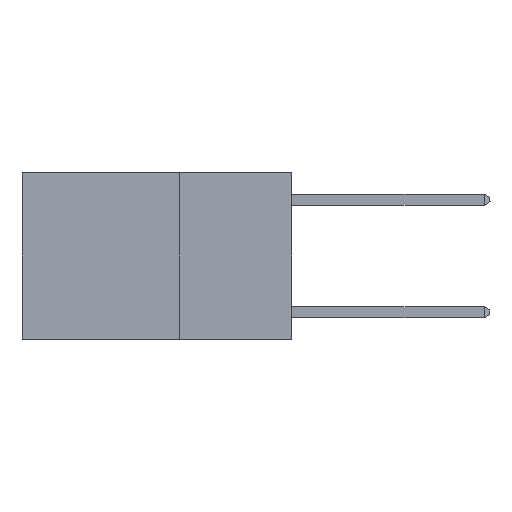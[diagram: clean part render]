
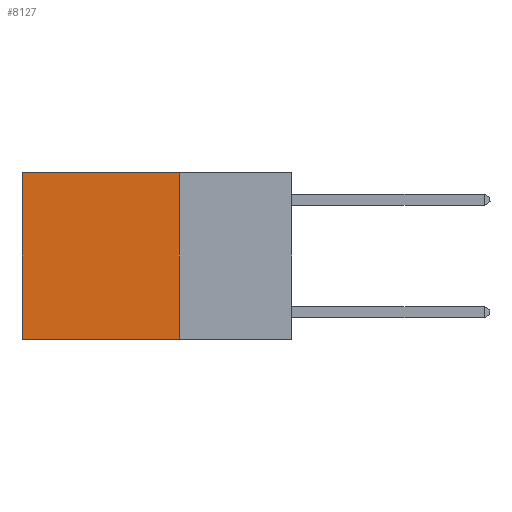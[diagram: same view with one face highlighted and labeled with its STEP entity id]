
A CAD part, left-side view. The second image highlights one B-rep face of the part: STEP entity #8127.
In plain terms, the highlighted planar face has unit normal (-1, 0, 0).
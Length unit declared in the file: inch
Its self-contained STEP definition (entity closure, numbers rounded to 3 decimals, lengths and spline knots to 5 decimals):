
#13 = CARTESIAN_POINT ( 'NONE',  ( 0.2625, 0.25, -0.37 ) ) ;
#69 = VERTEX_POINT ( 'NONE', #13 ) ;
#527 = CARTESIAN_POINT ( 'NONE',  ( 0.2625, 0.25, 0. ) ) ;
#608 = ORIENTED_EDGE ( 'NONE', *, *, #3062, .T. ) ;
#844 = EDGE_LOOP ( 'NONE', ( #2182, #7662, #9152, #608 ) ) ;
#1154 = VECTOR ( 'NONE', #4065, 39.37008 ) ;
#1278 = DIRECTION ( 'NONE',  ( 1., 0., 0. ) ) ;
#1807 = VECTOR ( 'NONE', #4570, 39.37008 ) ;
#2123 = CARTESIAN_POINT ( 'NONE',  ( 0.2625, 0.6, 0. ) ) ;
#2182 = ORIENTED_EDGE ( 'NONE', *, *, #4545, .T. ) ;
#2371 = CARTESIAN_POINT ( 'NONE',  ( 0.2625, 0.6, -0.37 ) ) ;
#2386 = FACE_OUTER_BOUND ( 'NONE', #844, .T. ) ;
#2499 = EDGE_CURVE ( 'NONE', #5500, #69, #8666, .T. ) ;
#3062 = EDGE_CURVE ( 'NONE', #5500, #7099, #7307, .T. ) ;
#4065 = DIRECTION ( 'NONE',  ( 0., 0., -1. ) ) ;
#4492 = PLANE ( 'NONE',  #6735 ) ;
#4545 = EDGE_CURVE ( 'NONE', #7099, #7263, #8053, .T. ) ;
#4570 = DIRECTION ( 'NONE',  ( 0., 1., 0. ) ) ;
#4842 = CARTESIAN_POINT ( 'NONE',  ( 0.2625, 0.25, 0. ) ) ;
#5004 = EDGE_CURVE ( 'NONE', #69, #7263, #7740, .T. ) ;
#5500 = VERTEX_POINT ( 'NONE', #9041 ) ;
#5644 = VECTOR ( 'NONE', #6610, 39.37008 ) ;
#5980 = CARTESIAN_POINT ( 'NONE',  ( 0.2625, 0.25, 0. ) ) ;
#6012 = CARTESIAN_POINT ( 'NONE',  ( 0.2625, 0.6, 0. ) ) ;
#6382 = VECTOR ( 'NONE', #7897, 39.37008 ) ;
#6522 = DIRECTION ( 'NONE',  ( 0., 0., -1. ) ) ;
#6610 = DIRECTION ( 'NONE',  ( 0., 1., 0. ) ) ;
#6735 = AXIS2_PLACEMENT_3D ( 'NONE', #527, #1278, #6522 ) ;
#7099 = VERTEX_POINT ( 'NONE', #2123 ) ;
#7174 = CARTESIAN_POINT ( 'NONE',  ( 0.2625, 0.25, -0.37 ) ) ;
#7263 = VERTEX_POINT ( 'NONE', #2371 ) ;
#7307 = LINE ( 'NONE', #5980, #5644 ) ;
#7662 = ORIENTED_EDGE ( 'NONE', *, *, #5004, .F. ) ;
#7740 = LINE ( 'NONE', #7174, #1807 ) ;
#7897 = DIRECTION ( 'NONE',  ( 0., 0., -1. ) ) ;
#8053 = LINE ( 'NONE', #6012, #6382 ) ;
#8127 = ADVANCED_FACE ( 'NONE', ( #2386 ), #4492, .F. ) ;
#8666 = LINE ( 'NONE', #4842, #1154 ) ;
#9041 = CARTESIAN_POINT ( 'NONE',  ( 0.2625, 0.25, 0. ) ) ;
#9152 = ORIENTED_EDGE ( 'NONE', *, *, #2499, .F. ) ;
